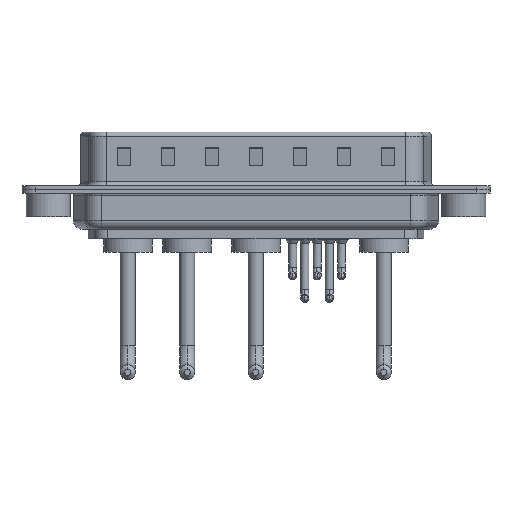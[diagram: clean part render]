
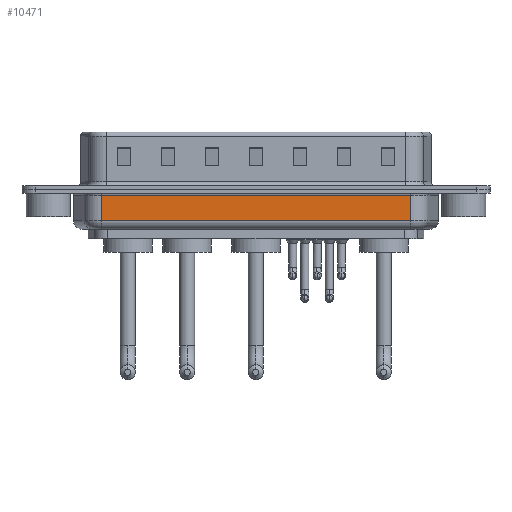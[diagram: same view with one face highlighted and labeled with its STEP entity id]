
A CAD part, front view. The second image highlights one B-rep face of the part: STEP entity #10471.
In plain terms, the highlighted planar face has unit normal (0, -1, 0).
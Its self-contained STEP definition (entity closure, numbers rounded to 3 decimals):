
#941 = CARTESIAN_POINT ( 'NONE',  ( 6.006, -5.35, -4.5 ) ) ;
#1500 = DIRECTION ( 'NONE',  ( 0., 0., 1. ) ) ;
#1567 = CARTESIAN_POINT ( 'NONE',  ( 6.006, -5.35, -3.5 ) ) ;
#2977 = AXIS2_PLACEMENT_3D ( 'NONE', #941, #13236, #13125 ) ;
#3252 = ORIENTED_EDGE ( 'NONE', *, *, #14853, .T. ) ;
#5506 = EDGE_CURVE ( 'NONE', #16267, #11279, #16584, .T. ) ;
#6292 = FACE_OUTER_BOUND ( 'NONE', #21221, .T. ) ;
#8734 = DIRECTION ( 'NONE',  ( -1., 0., 0. ) ) ;
#8959 = VERTEX_POINT ( 'NONE', #17664 ) ;
#10452 = VECTOR ( 'NONE', #15214, 1000. ) ;
#10471 = ADVANCED_FACE ( 'NONE', ( #6292 ), #18019, .F. ) ;
#10749 = ORIENTED_EDGE ( 'NONE', *, *, #17180, .T. ) ;
#11279 = VERTEX_POINT ( 'NONE', #17969 ) ;
#11859 = LINE ( 'NONE', #17085, #13266 ) ;
#13125 = DIRECTION ( 'NONE',  ( 0., 0., 1. ) ) ;
#13165 = CARTESIAN_POINT ( 'NONE',  ( 6.006, -5.35, -4.5 ) ) ;
#13236 = DIRECTION ( 'NONE',  ( 0., 1., 0. ) ) ;
#13266 = VECTOR ( 'NONE', #1500, 1000. ) ;
#13962 = VECTOR ( 'NONE', #19991, 1000. ) ;
#14250 = ORIENTED_EDGE ( 'NONE', *, *, #5506, .F. ) ;
#14853 = EDGE_CURVE ( 'NONE', #20105, #8959, #11859, .T. ) ;
#15214 = DIRECTION ( 'NONE',  ( 1., 0., 0. ) ) ;
#16267 = VERTEX_POINT ( 'NONE', #21164 ) ;
#16584 = LINE ( 'NONE', #13165, #13962 ) ;
#16597 = VECTOR ( 'NONE', #8734, 1000. ) ;
#17085 = CARTESIAN_POINT ( 'NONE',  ( 41.044, -5.35, -4.5 ) ) ;
#17180 = EDGE_CURVE ( 'NONE', #8959, #11279, #17599, .T. ) ;
#17599 = LINE ( 'NONE', #20879, #16597 ) ;
#17664 = CARTESIAN_POINT ( 'NONE',  ( 41.044, -5.35, -0.65 ) ) ;
#17969 = CARTESIAN_POINT ( 'NONE',  ( 6.006, -5.35, -0.65 ) ) ;
#18019 = PLANE ( 'NONE',  #2977 ) ;
#18846 = LINE ( 'NONE', #1567, #10452 ) ;
#19395 = EDGE_CURVE ( 'NONE', #16267, #20105, #18846, .T. ) ;
#19991 = DIRECTION ( 'NONE',  ( 0., 0., 1. ) ) ;
#20051 = ORIENTED_EDGE ( 'NONE', *, *, #19395, .T. ) ;
#20105 = VERTEX_POINT ( 'NONE', #21413 ) ;
#20879 = CARTESIAN_POINT ( 'NONE',  ( 6.006, -5.35, -0.65 ) ) ;
#21164 = CARTESIAN_POINT ( 'NONE',  ( 6.006, -5.35, -3.5 ) ) ;
#21221 = EDGE_LOOP ( 'NONE', ( #14250, #20051, #3252, #10749 ) ) ;
#21413 = CARTESIAN_POINT ( 'NONE',  ( 41.044, -5.35, -3.5 ) ) ;
